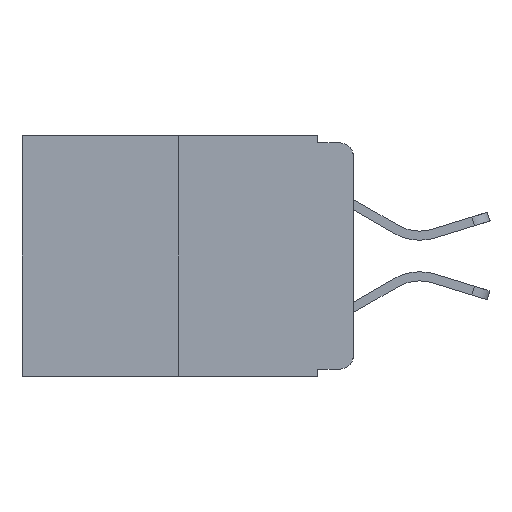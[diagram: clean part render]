
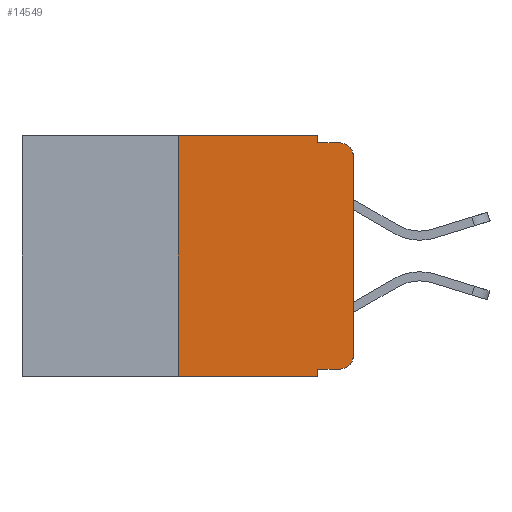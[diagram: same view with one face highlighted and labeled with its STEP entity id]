
A CAD part, left-side view. The second image highlights one B-rep face of the part: STEP entity #14549.
In plain terms, the highlighted planar face has unit normal (-1, 0, 0).
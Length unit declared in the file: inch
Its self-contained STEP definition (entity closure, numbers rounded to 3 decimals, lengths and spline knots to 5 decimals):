
#10 = CARTESIAN_POINT ( 'NONE',  ( 0., 0.051, -0.343 ) ) ;
#735 = CARTESIAN_POINT ( 'NONE',  ( 0., 0.473, 0. ) ) ;
#828 = VECTOR ( 'NONE', #16644, 39.37008 ) ;
#854 = CARTESIAN_POINT ( 'NONE',  ( 0., 0., -0.03 ) ) ;
#863 = VERTEX_POINT ( 'NONE', #881 ) ;
#866 = VERTEX_POINT ( 'NONE', #854 ) ;
#881 = CARTESIAN_POINT ( 'NONE',  ( 0., 0.25, 0. ) ) ;
#983 = VERTEX_POINT ( 'NONE', #11410 ) ;
#992 = EDGE_CURVE ( 'NONE', #13723, #866, #15811, .T. ) ;
#1533 = EDGE_CURVE ( 'NONE', #3698, #2267, #19281, .T. ) ;
#1657 = AXIS2_PLACEMENT_3D ( 'NONE', #735, #18669, #8084 ) ;
#2267 = VERTEX_POINT ( 'NONE', #5443 ) ;
#3407 = AXIS2_PLACEMENT_3D ( 'NONE', #15895, #5127, #17633 ) ;
#3445 = EDGE_LOOP ( 'NONE', ( #10132, #10450, #13268, #3580, #5512, #5875, #21789, #3881, #7694, #7923 ) ) ;
#3580 = ORIENTED_EDGE ( 'NONE', *, *, #10966, .F. ) ;
#3698 = VERTEX_POINT ( 'NONE', #10618 ) ;
#3881 = ORIENTED_EDGE ( 'NONE', *, *, #5534, .F. ) ;
#4272 = LINE ( 'NONE', #17722, #13337 ) ;
#4383 = CARTESIAN_POINT ( 'NONE',  ( 0., 0.25, 0. ) ) ;
#4458 = CARTESIAN_POINT ( 'NONE',  ( 0., 0.051, -0.01 ) ) ;
#4555 = LINE ( 'NONE', #4383, #14704 ) ;
#4647 = EDGE_CURVE ( 'NONE', #5224, #16761, #15472, .T. ) ;
#5020 = FACE_OUTER_BOUND ( 'NONE', #3445, .T. ) ;
#5127 = DIRECTION ( 'NONE',  ( -1., 0., 0. ) ) ;
#5224 = VERTEX_POINT ( 'NONE', #9767 ) ;
#5352 = VECTOR ( 'NONE', #8298, 39.37008 ) ;
#5443 = CARTESIAN_POINT ( 'NONE',  ( 0., 0.02, -0.333 ) ) ;
#5512 = ORIENTED_EDGE ( 'NONE', *, *, #11459, .F. ) ;
#5534 = EDGE_CURVE ( 'NONE', #3698, #11555, #16283, .T. ) ;
#5875 = ORIENTED_EDGE ( 'NONE', *, *, #19346, .F. ) ;
#6239 = DIRECTION ( 'NONE',  ( 0., 0., 1. ) ) ;
#6782 = VECTOR ( 'NONE', #7079, 39.37008 ) ;
#7079 = DIRECTION ( 'NONE',  ( 0., 0., -1. ) ) ;
#7131 = DIRECTION ( 'NONE',  ( -1., 0., 0. ) ) ;
#7559 = CARTESIAN_POINT ( 'NONE',  ( 0., 0.051, 0. ) ) ;
#7694 = ORIENTED_EDGE ( 'NONE', *, *, #1533, .T. ) ;
#7923 = ORIENTED_EDGE ( 'NONE', *, *, #18919, .T. ) ;
#8084 = DIRECTION ( 'NONE',  ( 0., 0., -1. ) ) ;
#8298 = DIRECTION ( 'NONE',  ( 0., -1., 0. ) ) ;
#8740 = VECTOR ( 'NONE', #13411, 39.37008 ) ;
#9767 = CARTESIAN_POINT ( 'NONE',  ( 0., 0.051, -0.01 ) ) ;
#10132 = ORIENTED_EDGE ( 'NONE', *, *, #992, .T. ) ;
#10450 = ORIENTED_EDGE ( 'NONE', *, *, #15309, .T. ) ;
#10529 = VECTOR ( 'NONE', #22829, 39.37008 ) ;
#10618 = CARTESIAN_POINT ( 'NONE',  ( 0., 0.051, -0.333 ) ) ;
#10829 = VECTOR ( 'NONE', #19866, 39.37008 ) ;
#10852 = CARTESIAN_POINT ( 'NONE',  ( 0., 0., 0. ) ) ;
#10966 = EDGE_CURVE ( 'NONE', #983, #5224, #14458, .T. ) ;
#11103 = CARTESIAN_POINT ( 'NONE',  ( 0., 0., -0.313 ) ) ;
#11410 = CARTESIAN_POINT ( 'NONE',  ( 0., 0.051, 0. ) ) ;
#11459 = EDGE_CURVE ( 'NONE', #863, #983, #4272, .T. ) ;
#11555 = VERTEX_POINT ( 'NONE', #10 ) ;
#12916 = AXIS2_PLACEMENT_3D ( 'NONE', #17788, #7131, #19478 ) ;
#13268 = ORIENTED_EDGE ( 'NONE', *, *, #4647, .F. ) ;
#13337 = VECTOR ( 'NONE', #19424, 39.37008 ) ;
#13411 = DIRECTION ( 'NONE',  ( 0., -1., 0. ) ) ;
#13437 = PLANE ( 'NONE',  #1657 ) ;
#13508 = LINE ( 'NONE', #21931, #8740 ) ;
#13723 = VERTEX_POINT ( 'NONE', #11103 ) ;
#14458 = LINE ( 'NONE', #7559, #10829 ) ;
#14549 = ADVANCED_FACE ( 'NONE', ( #5020 ), #13437, .F. ) ;
#14704 = VECTOR ( 'NONE', #6239, 39.37008 ) ;
#15309 = EDGE_CURVE ( 'NONE', #866, #16761, #20723, .T. ) ;
#15472 = LINE ( 'NONE', #4458, #5352 ) ;
#15811 = LINE ( 'NONE', #10852, #10529 ) ;
#15892 = VERTEX_POINT ( 'NONE', #19236 ) ;
#15895 = CARTESIAN_POINT ( 'NONE',  ( 0., 0.02, -0.313 ) ) ;
#15977 = CARTESIAN_POINT ( 'NONE',  ( 0., 0.051, 0. ) ) ;
#16283 = LINE ( 'NONE', #15977, #6782 ) ;
#16644 = DIRECTION ( 'NONE',  ( 0., -1., 0. ) ) ;
#16761 = VERTEX_POINT ( 'NONE', #18173 ) ;
#17631 = CARTESIAN_POINT ( 'NONE',  ( 0., 0.051, -0.333 ) ) ;
#17633 = DIRECTION ( 'NONE',  ( 0., 0., -1. ) ) ;
#17722 = CARTESIAN_POINT ( 'NONE',  ( 0., 0.473, 0. ) ) ;
#17788 = CARTESIAN_POINT ( 'NONE',  ( 0., 0.02, -0.03 ) ) ;
#18173 = CARTESIAN_POINT ( 'NONE',  ( 0., 0.02, -0.01 ) ) ;
#18669 = DIRECTION ( 'NONE',  ( 1., 0., 0. ) ) ;
#18796 = CIRCLE ( 'NONE', #3407, 0.02 ) ;
#18919 = EDGE_CURVE ( 'NONE', #2267, #13723, #18796, .T. ) ;
#19236 = CARTESIAN_POINT ( 'NONE',  ( 0., 0.25, -0.343 ) ) ;
#19281 = LINE ( 'NONE', #17631, #828 ) ;
#19346 = EDGE_CURVE ( 'NONE', #15892, #863, #4555, .T. ) ;
#19424 = DIRECTION ( 'NONE',  ( 0., -1., 0. ) ) ;
#19478 = DIRECTION ( 'NONE',  ( 0., 0., -1. ) ) ;
#19866 = DIRECTION ( 'NONE',  ( 0., 0., -1. ) ) ;
#20723 = CIRCLE ( 'NONE', #12916, 0.02 ) ;
#21488 = EDGE_CURVE ( 'NONE', #15892, #11555, #13508, .T. ) ;
#21789 = ORIENTED_EDGE ( 'NONE', *, *, #21488, .T. ) ;
#21931 = CARTESIAN_POINT ( 'NONE',  ( 0., 0.473, -0.343 ) ) ;
#22829 = DIRECTION ( 'NONE',  ( 0., 0., 1. ) ) ;
